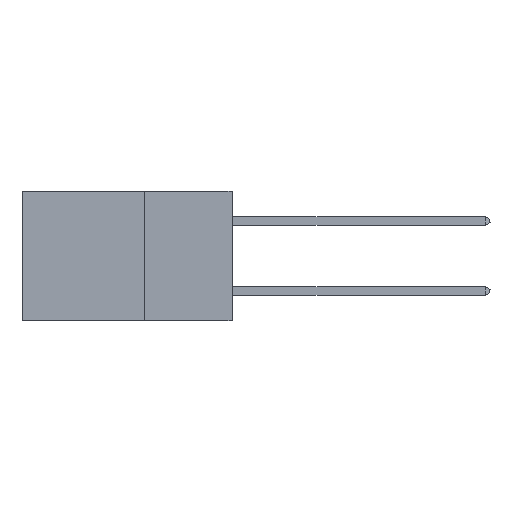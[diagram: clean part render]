
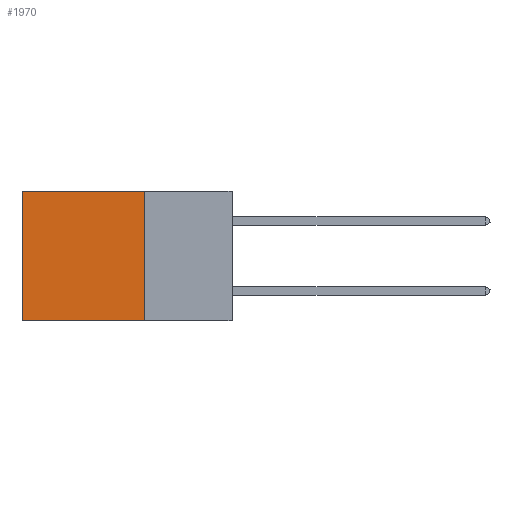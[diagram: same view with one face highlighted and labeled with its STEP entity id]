
A CAD part, left-side view. The second image highlights one B-rep face of the part: STEP entity #1970.
In plain terms, the highlighted planar face has unit normal (-1, 0, 0).
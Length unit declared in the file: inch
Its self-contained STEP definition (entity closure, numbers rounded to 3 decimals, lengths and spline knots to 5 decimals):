
#79 = DIRECTION ( 'NONE',  ( 0., 1., 0. ) ) ;
#83 = VERTEX_POINT ( 'NONE', #3369 ) ;
#162 = VECTOR ( 'NONE', #25160, 39.37008 ) ;
#492 = AXIS2_PLACEMENT_3D ( 'NONE', #20944, #16225, #1292 ) ;
#545 = VECTOR ( 'NONE', #79, 39.37008 ) ;
#1292 = DIRECTION ( 'NONE',  ( 0., 0., -1. ) ) ;
#1692 = EDGE_LOOP ( 'NONE', ( #19291, #16291, #22681, #31736 ) ) ;
#1970 = ADVANCED_FACE ( 'NONE', ( #27452 ), #13718, .F. ) ;
#2733 = VERTEX_POINT ( 'NONE', #9450 ) ;
#3369 = CARTESIAN_POINT ( 'NONE',  ( 0.2875, 0.25, 0. ) ) ;
#3521 = EDGE_CURVE ( 'NONE', #2733, #14745, #27333, .T. ) ;
#3632 = DIRECTION ( 'NONE',  ( 0., 1., 0. ) ) ;
#4664 = CARTESIAN_POINT ( 'NONE',  ( 0.2875, 0.25, -0.37 ) ) ;
#5307 = CARTESIAN_POINT ( 'NONE',  ( 0.2875, 0.6, 0. ) ) ;
#6779 = EDGE_CURVE ( 'NONE', #83, #16641, #22075, .T. ) ;
#7561 = CARTESIAN_POINT ( 'NONE',  ( 0.2875, 0.25, 0. ) ) ;
#8053 = DIRECTION ( 'NONE',  ( 0., 0., -1. ) ) ;
#9450 = CARTESIAN_POINT ( 'NONE',  ( 0.2875, 0.25, -0.37 ) ) ;
#13718 = PLANE ( 'NONE',  #492 ) ;
#14745 = VERTEX_POINT ( 'NONE', #15177 ) ;
#15177 = CARTESIAN_POINT ( 'NONE',  ( 0.2875, 0.6, -0.37 ) ) ;
#16225 = DIRECTION ( 'NONE',  ( 1., 0., 0. ) ) ;
#16291 = ORIENTED_EDGE ( 'NONE', *, *, #3521, .F. ) ;
#16641 = VERTEX_POINT ( 'NONE', #29933 ) ;
#19291 = ORIENTED_EDGE ( 'NONE', *, *, #27195, .T. ) ;
#20069 = CARTESIAN_POINT ( 'NONE',  ( 0.2875, 0.25, 0. ) ) ;
#20944 = CARTESIAN_POINT ( 'NONE',  ( 0.2875, 0.25, 0. ) ) ;
#22075 = LINE ( 'NONE', #20069, #545 ) ;
#22681 = ORIENTED_EDGE ( 'NONE', *, *, #29107, .F. ) ;
#25160 = DIRECTION ( 'NONE',  ( 0., 0., -1. ) ) ;
#27195 = EDGE_CURVE ( 'NONE', #16641, #14745, #31953, .T. ) ;
#27333 = LINE ( 'NONE', #4664, #28876 ) ;
#27452 = FACE_OUTER_BOUND ( 'NONE', #1692, .T. ) ;
#28876 = VECTOR ( 'NONE', #3632, 39.37008 ) ;
#29107 = EDGE_CURVE ( 'NONE', #83, #2733, #30661, .T. ) ;
#29933 = CARTESIAN_POINT ( 'NONE',  ( 0.2875, 0.6, 0. ) ) ;
#30362 = VECTOR ( 'NONE', #8053, 39.37008 ) ;
#30661 = LINE ( 'NONE', #7561, #162 ) ;
#31736 = ORIENTED_EDGE ( 'NONE', *, *, #6779, .T. ) ;
#31953 = LINE ( 'NONE', #5307, #30362 ) ;
